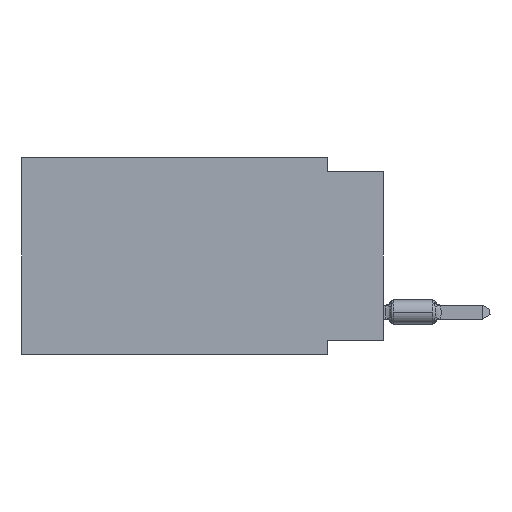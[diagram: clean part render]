
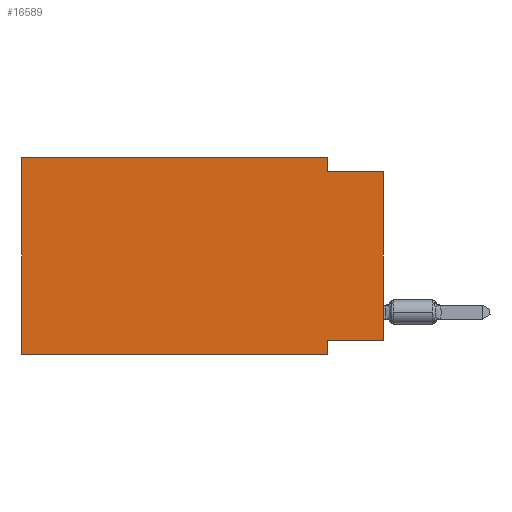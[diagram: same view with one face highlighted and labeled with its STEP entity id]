
A CAD part, left-side view. The second image highlights one B-rep face of the part: STEP entity #16589.
In plain terms, the highlighted planar face has unit normal (-1, 0, 0).
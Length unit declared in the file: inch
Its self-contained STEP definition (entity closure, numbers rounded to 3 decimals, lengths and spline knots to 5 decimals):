
#8623 = ORIENTED_EDGE ( 'NONE', *, *, #68817, .F. ) ;
#10403 = DIRECTION ( 'NONE',  ( 1., 0., 0. ) ) ;
#10830 = DIRECTION ( 'NONE',  ( 0., 0., -1. ) ) ;
#13084 = CARTESIAN_POINT ( 'NONE',  ( 0., 0., 0. ) ) ;
#15051 = CARTESIAN_POINT ( 'NONE',  ( 0., 0.645, 0. ) ) ;
#15095 = CARTESIAN_POINT ( 'NONE',  ( 0., 0.645, 0. ) ) ;
#16589 = ADVANCED_FACE ( 'NONE', ( #75683 ), #74289, .F. ) ;
#18188 = VECTOR ( 'NONE', #20442, 39.37008 ) ;
#20442 = DIRECTION ( 'NONE',  ( 0., -1., 0. ) ) ;
#22155 = LINE ( 'NONE', #15051, #42290 ) ;
#24900 = CARTESIAN_POINT ( 'NONE',  ( 0., 0., -0.325 ) ) ;
#25560 = VERTEX_POINT ( 'NONE', #15095 ) ;
#26049 = CARTESIAN_POINT ( 'NONE',  ( 0., 0.1, -0.025 ) ) ;
#32312 = EDGE_CURVE ( 'NONE', #25560, #78851, #36212, .T. ) ;
#33024 = LINE ( 'NONE', #85060, #91314 ) ;
#33531 = LINE ( 'NONE', #41095, #72096 ) ;
#34058 = VERTEX_POINT ( 'NONE', #60474 ) ;
#35890 = CARTESIAN_POINT ( 'NONE',  ( 0., 0.1, 0. ) ) ;
#35956 = CARTESIAN_POINT ( 'NONE',  ( 0., 0.1, -0.35 ) ) ;
#36212 = LINE ( 'NONE', #50876, #64749 ) ;
#38605 = VECTOR ( 'NONE', #39554, 39.37008 ) ;
#39546 = VERTEX_POINT ( 'NONE', #67682 ) ;
#39554 = DIRECTION ( 'NONE',  ( 0., 1., 0. ) ) ;
#39719 = DIRECTION ( 'NONE',  ( 0., 0., -1. ) ) ;
#40321 = EDGE_CURVE ( 'NONE', #73775, #40818, #64439, .T. ) ;
#40818 = VERTEX_POINT ( 'NONE', #35956 ) ;
#41095 = CARTESIAN_POINT ( 'NONE',  ( 0., 0.1, -0.35 ) ) ;
#41161 = CARTESIAN_POINT ( 'NONE',  ( 0., 0.1, -0.325 ) ) ;
#42290 = VECTOR ( 'NONE', #43936, 39.37008 ) ;
#42849 = DIRECTION ( 'NONE',  ( 0., -1., 0. ) ) ;
#43219 = ORIENTED_EDGE ( 'NONE', *, *, #83723, .F. ) ;
#43936 = DIRECTION ( 'NONE',  ( 0., 0., 1. ) ) ;
#45583 = VECTOR ( 'NONE', #57359, 39.37008 ) ;
#48902 = VECTOR ( 'NONE', #72214, 39.37008 ) ;
#50726 = LINE ( 'NONE', #72952, #45583 ) ;
#50876 = CARTESIAN_POINT ( 'NONE',  ( 0., 0.645, 0. ) ) ;
#52473 = VERTEX_POINT ( 'NONE', #26049 ) ;
#52819 = EDGE_LOOP ( 'NONE', ( #61841, #8623, #84315, #84032, #74151, #93632, #43219, #84287 ) ) ;
#56177 = DIRECTION ( 'NONE',  ( 0., -1., 0. ) ) ;
#57359 = DIRECTION ( 'NONE',  ( 0., 0., -1. ) ) ;
#59498 = EDGE_CURVE ( 'NONE', #78851, #52473, #50726, .T. ) ;
#60474 = CARTESIAN_POINT ( 'NONE',  ( 0., 0., -0.025 ) ) ;
#60869 = EDGE_CURVE ( 'NONE', #73775, #25560, #22155, .T. ) ;
#61841 = ORIENTED_EDGE ( 'NONE', *, *, #87365, .T. ) ;
#64439 = LINE ( 'NONE', #78652, #18188 ) ;
#64749 = VECTOR ( 'NONE', #42849, 39.37008 ) ;
#67017 = LINE ( 'NONE', #24900, #38605 ) ;
#67682 = CARTESIAN_POINT ( 'NONE',  ( 0., 0., -0.325 ) ) ;
#68473 = VERTEX_POINT ( 'NONE', #41161 ) ;
#68817 = EDGE_CURVE ( 'NONE', #52473, #34058, #33024, .T. ) ;
#70361 = EDGE_CURVE ( 'NONE', #39546, #68473, #67017, .T. ) ;
#72096 = VECTOR ( 'NONE', #10830, 39.37008 ) ;
#72214 = DIRECTION ( 'NONE',  ( 0., 0., 1. ) ) ;
#72520 = CARTESIAN_POINT ( 'NONE',  ( 0., 0.645, -0.35 ) ) ;
#72952 = CARTESIAN_POINT ( 'NONE',  ( 0., 0.1, 0. ) ) ;
#73775 = VERTEX_POINT ( 'NONE', #72520 ) ;
#74151 = ORIENTED_EDGE ( 'NONE', *, *, #60869, .F. ) ;
#74289 = PLANE ( 'NONE',  #74513 ) ;
#74513 = AXIS2_PLACEMENT_3D ( 'NONE', #88988, #10403, #39719 ) ;
#75683 = FACE_OUTER_BOUND ( 'NONE', #52819, .T. ) ;
#78652 = CARTESIAN_POINT ( 'NONE',  ( 0., 0.645, -0.35 ) ) ;
#78851 = VERTEX_POINT ( 'NONE', #35890 ) ;
#83723 = EDGE_CURVE ( 'NONE', #68473, #40818, #33531, .T. ) ;
#84032 = ORIENTED_EDGE ( 'NONE', *, *, #32312, .F. ) ;
#84287 = ORIENTED_EDGE ( 'NONE', *, *, #70361, .F. ) ;
#84315 = ORIENTED_EDGE ( 'NONE', *, *, #59498, .F. ) ;
#85060 = CARTESIAN_POINT ( 'NONE',  ( 0., 0., -0.025 ) ) ;
#86434 = LINE ( 'NONE', #13084, #48902 ) ;
#87365 = EDGE_CURVE ( 'NONE', #39546, #34058, #86434, .T. ) ;
#88988 = CARTESIAN_POINT ( 'NONE',  ( 0., 0.645, 0. ) ) ;
#91314 = VECTOR ( 'NONE', #56177, 39.37008 ) ;
#93632 = ORIENTED_EDGE ( 'NONE', *, *, #40321, .T. ) ;
